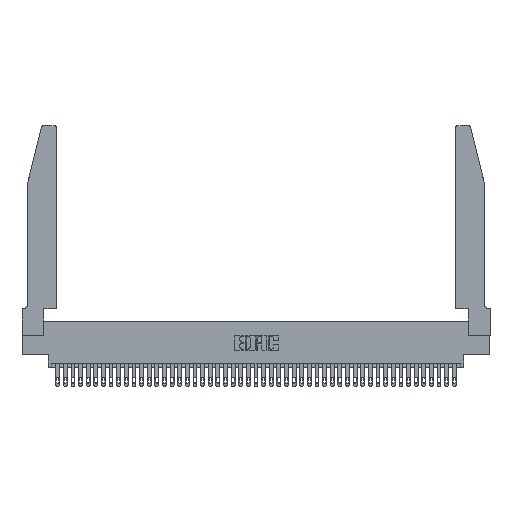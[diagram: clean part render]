
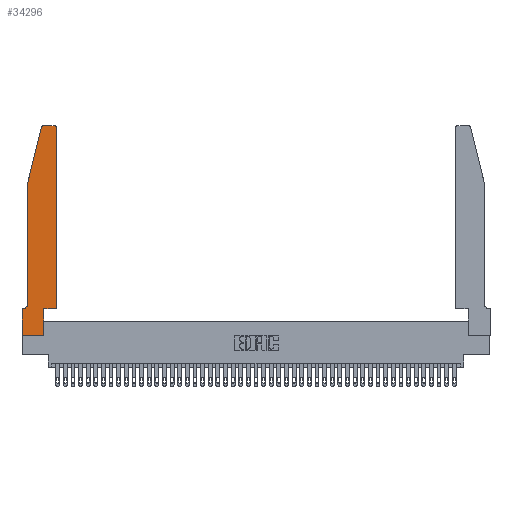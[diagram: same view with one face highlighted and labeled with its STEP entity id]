
A CAD part, top view. The second image highlights one B-rep face of the part: STEP entity #34296.
In plain terms, the highlighted planar face has unit normal (0, 0, 1).
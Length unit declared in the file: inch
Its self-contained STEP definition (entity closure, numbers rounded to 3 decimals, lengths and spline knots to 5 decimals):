
#124 = FACE_OUTER_BOUND ( 'NONE', #14156, .T. ) ;
#488 = VERTEX_POINT ( 'NONE', #3574 ) ;
#854 = CARTESIAN_POINT ( 'NONE',  ( 0.0755, 0.42, 0.37 ) ) ;
#1359 = DIRECTION ( 'NONE',  ( 1., 0., 0. ) ) ;
#1383 = PLANE ( 'NONE',  #6746 ) ;
#1548 = DIRECTION ( 'NONE',  ( -1., 0., 0. ) ) ;
#3192 = LINE ( 'NONE', #33151, #13488 ) ;
#3269 = EDGE_CURVE ( 'NONE', #12064, #7476, #34351, .T. ) ;
#3574 = CARTESIAN_POINT ( 'NONE',  ( 0.25487, 2.72718, 0.37 ) ) ;
#3660 = ORIENTED_EDGE ( 'NONE', *, *, #24299, .T. ) ;
#4728 = DIRECTION ( 'NONE',  ( 0., 0., 1. ) ) ;
#5564 = LINE ( 'NONE', #35903, #41457 ) ;
#6746 = AXIS2_PLACEMENT_3D ( 'NONE', #21835, #4728, #15210 ) ;
#7302 = CIRCLE ( 'NONE', #13008, 0.07 ) ;
#7476 = VERTEX_POINT ( 'NONE', #12057 ) ;
#7672 = VECTOR ( 'NONE', #30003, 39.37008 ) ;
#7731 = CARTESIAN_POINT ( 'NONE',  ( 0.284, 2.72, 0.37 ) ) ;
#7772 = LINE ( 'NONE', #24753, #9998 ) ;
#8500 = CARTESIAN_POINT ( 'NONE',  ( 0.2865, 0.35, 0.37 ) ) ;
#8808 = EDGE_CURVE ( 'NONE', #7476, #26364, #15051, .T. ) ;
#8984 = CARTESIAN_POINT ( 'NONE',  ( 0.4205, 2.72, 0.37 ) ) ;
#9175 = ORIENTED_EDGE ( 'NONE', *, *, #43222, .T. ) ;
#9670 = AXIS2_PLACEMENT_3D ( 'NONE', #8984, #37236, #19393 ) ;
#9998 = VECTOR ( 'NONE', #25052, 39.37008 ) ;
#11610 = CARTESIAN_POINT ( 'NONE',  ( 0.0755, 2., 0.37 ) ) ;
#11899 = CIRCLE ( 'NONE', #27239, 0.03 ) ;
#11976 = EDGE_CURVE ( 'NONE', #22715, #22635, #5564, .T. ) ;
#12028 = EDGE_CURVE ( 'NONE', #488, #16610, #32124, .T. ) ;
#12057 = CARTESIAN_POINT ( 'NONE',  ( 0.2865, 0., 0.37 ) ) ;
#12064 = VERTEX_POINT ( 'NONE', #16346 ) ;
#12727 = VERTEX_POINT ( 'NONE', #39486 ) ;
#12926 = EDGE_CURVE ( 'NONE', #12727, #17185, #29918, .T. ) ;
#13008 = AXIS2_PLACEMENT_3D ( 'NONE', #44904, #20690, #17221 ) ;
#13082 = CARTESIAN_POINT ( 'NONE',  ( 0., 0., 0.37 ) ) ;
#13167 = VECTOR ( 'NONE', #19418, 39.37008 ) ;
#13488 = VECTOR ( 'NONE', #1548, 39.37008 ) ;
#13854 = VERTEX_POINT ( 'NONE', #24978 ) ;
#14156 = EDGE_LOOP ( 'NONE', ( #22522, #38190, #19922, #34958, #23140, #42641, #9175, #25307, #37985, #3660, #30208, #23797 ) ) ;
#14334 = VECTOR ( 'NONE', #27370, 39.37008 ) ;
#14553 = CARTESIAN_POINT ( 'NONE',  ( 0.4505, 0.35, 0.37 ) ) ;
#15051 = LINE ( 'NONE', #8500, #41749 ) ;
#15210 = DIRECTION ( 'NONE',  ( 1., 0., 0. ) ) ;
#16346 = CARTESIAN_POINT ( 'NONE',  ( 0., 0., 0.37 ) ) ;
#16610 = VERTEX_POINT ( 'NONE', #11610 ) ;
#17185 = VERTEX_POINT ( 'NONE', #26812 ) ;
#17221 = DIRECTION ( 'NONE',  ( -1., 0., 0. ) ) ;
#17223 = CARTESIAN_POINT ( 'NONE',  ( 0.0755, 2., 0.37 ) ) ;
#18350 = CARTESIAN_POINT ( 'NONE',  ( 0.0055, 0.35, 0.37 ) ) ;
#19393 = DIRECTION ( 'NONE',  ( 1., 0., 0. ) ) ;
#19418 = DIRECTION ( 'NONE',  ( 1., 0., 0. ) ) ;
#19922 = ORIENTED_EDGE ( 'NONE', *, *, #12028, .T. ) ;
#20008 = LINE ( 'NONE', #14553, #22730 ) ;
#20690 = DIRECTION ( 'NONE',  ( 0., 0., -1. ) ) ;
#21367 = EDGE_CURVE ( 'NONE', #16610, #40971, #7772, .T. ) ;
#21835 = CARTESIAN_POINT ( 'NONE',  ( 0., 0.35, 0.37 ) ) ;
#22522 = ORIENTED_EDGE ( 'NONE', *, *, #40606, .T. ) ;
#22619 = CARTESIAN_POINT ( 'NONE',  ( 0.284, 2.75, 0.37 ) ) ;
#22635 = VERTEX_POINT ( 'NONE', #39078 ) ;
#22715 = VERTEX_POINT ( 'NONE', #18350 ) ;
#22730 = VECTOR ( 'NONE', #1359, 39.37008 ) ;
#23040 = LINE ( 'NONE', #13082, #14334 ) ;
#23140 = ORIENTED_EDGE ( 'NONE', *, *, #27469, .T. ) ;
#23430 = DIRECTION ( 'NONE',  ( -1., 0., 0. ) ) ;
#23797 = ORIENTED_EDGE ( 'NONE', *, *, #12926, .T. ) ;
#24113 = EDGE_CURVE ( 'NONE', #36230, #488, #11899, .T. ) ;
#24299 = EDGE_CURVE ( 'NONE', #26364, #13854, #20008, .T. ) ;
#24753 = CARTESIAN_POINT ( 'NONE',  ( 0.0755, 2., 0.37 ) ) ;
#24978 = CARTESIAN_POINT ( 'NONE',  ( 0.4505, 0.35, 0.37 ) ) ;
#25052 = DIRECTION ( 'NONE',  ( 0., -1., 0. ) ) ;
#25307 = ORIENTED_EDGE ( 'NONE', *, *, #3269, .T. ) ;
#26364 = VERTEX_POINT ( 'NONE', #43401 ) ;
#26812 = CARTESIAN_POINT ( 'NONE',  ( 0.4205, 2.75, 0.37 ) ) ;
#27239 = AXIS2_PLACEMENT_3D ( 'NONE', #7731, #32169, #42243 ) ;
#27370 = DIRECTION ( 'NONE',  ( 0., -1., 0. ) ) ;
#27469 = EDGE_CURVE ( 'NONE', #40971, #22715, #7302, .T. ) ;
#29918 = CIRCLE ( 'NONE', #9670, 0.03 ) ;
#30003 = DIRECTION ( 'NONE',  ( 0., 1., 0. ) ) ;
#30208 = ORIENTED_EDGE ( 'NONE', *, *, #44521, .T. ) ;
#32124 = LINE ( 'NONE', #17223, #44198 ) ;
#32169 = DIRECTION ( 'NONE',  ( 0., 0., 1. ) ) ;
#32877 = CARTESIAN_POINT ( 'NONE',  ( 0.4505, 0.35, 0.37 ) ) ;
#33151 = CARTESIAN_POINT ( 'NONE',  ( 0.2605, 2.75, 0.37 ) ) ;
#34296 = ADVANCED_FACE ( 'NONE', ( #124 ), #1383, .T. ) ;
#34351 = LINE ( 'NONE', #43653, #13167 ) ;
#34958 = ORIENTED_EDGE ( 'NONE', *, *, #21367, .T. ) ;
#35903 = CARTESIAN_POINT ( 'NONE',  ( 0.0755, 0.35, 0.37 ) ) ;
#36230 = VERTEX_POINT ( 'NONE', #22619 ) ;
#37236 = DIRECTION ( 'NONE',  ( 0., 0., 1. ) ) ;
#37985 = ORIENTED_EDGE ( 'NONE', *, *, #8808, .T. ) ;
#38190 = ORIENTED_EDGE ( 'NONE', *, *, #24113, .T. ) ;
#39078 = CARTESIAN_POINT ( 'NONE',  ( 0., 0.35, 0.37 ) ) ;
#39486 = CARTESIAN_POINT ( 'NONE',  ( 0.4505, 2.72, 0.37 ) ) ;
#39957 = DIRECTION ( 'NONE',  ( 0., 1., 0. ) ) ;
#40606 = EDGE_CURVE ( 'NONE', #17185, #36230, #3192, .T. ) ;
#40971 = VERTEX_POINT ( 'NONE', #854 ) ;
#41273 = DIRECTION ( 'NONE',  ( -0.239, -0.971, 0. ) ) ;
#41442 = LINE ( 'NONE', #32877, #7672 ) ;
#41457 = VECTOR ( 'NONE', #23430, 39.37008 ) ;
#41749 = VECTOR ( 'NONE', #39957, 39.37008 ) ;
#42243 = DIRECTION ( 'NONE',  ( 1., 0., 0. ) ) ;
#42641 = ORIENTED_EDGE ( 'NONE', *, *, #11976, .T. ) ;
#43222 = EDGE_CURVE ( 'NONE', #22635, #12064, #23040, .T. ) ;
#43401 = CARTESIAN_POINT ( 'NONE',  ( 0.2865, 0.35, 0.37 ) ) ;
#43653 = CARTESIAN_POINT ( 'NONE',  ( 0., 0., 0.37 ) ) ;
#44198 = VECTOR ( 'NONE', #41273, 39.37008 ) ;
#44521 = EDGE_CURVE ( 'NONE', #13854, #12727, #41442, .T. ) ;
#44904 = CARTESIAN_POINT ( 'NONE',  ( 0.0055, 0.42, 0.37 ) ) ;
